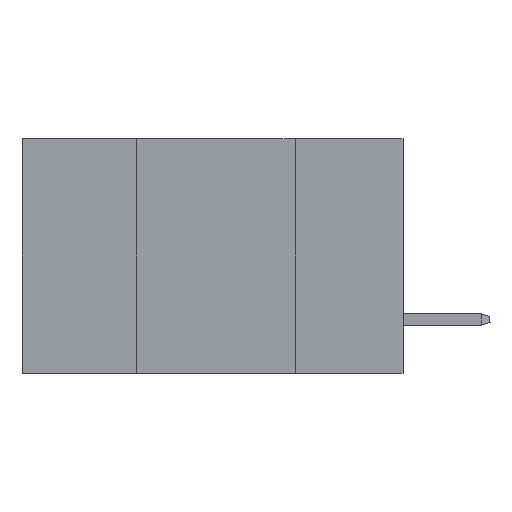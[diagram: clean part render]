
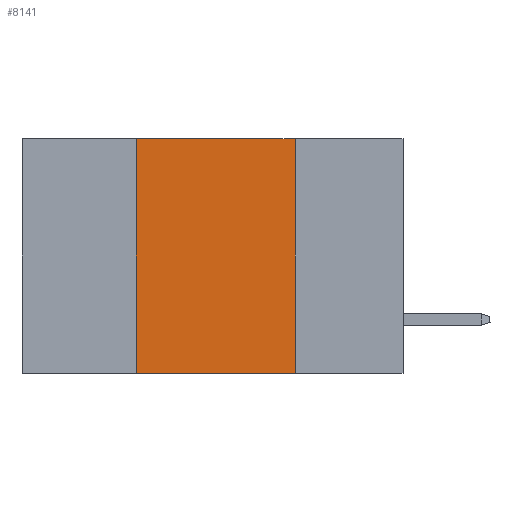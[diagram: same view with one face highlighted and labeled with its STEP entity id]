
A CAD part, left-side view. The second image highlights one B-rep face of the part: STEP entity #8141.
In plain terms, the highlighted planar face has unit normal (-1, 0, 0).
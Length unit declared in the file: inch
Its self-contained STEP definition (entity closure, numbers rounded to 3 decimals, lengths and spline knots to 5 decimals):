
#665 = VECTOR ( 'NONE', #13908, 39.37008 ) ;
#1241 = CARTESIAN_POINT ( 'NONE',  ( 0., 0.6, -0.37 ) ) ;
#1334 = LINE ( 'NONE', #2903, #665 ) ;
#1686 = DIRECTION ( 'NONE',  ( 0., 0., -1. ) ) ;
#1726 = VECTOR ( 'NONE', #15344, 39.37008 ) ;
#2518 = LINE ( 'NONE', #16546, #1726 ) ;
#2889 = ORIENTED_EDGE ( 'NONE', *, *, #7016, .F. ) ;
#2903 = CARTESIAN_POINT ( 'NONE',  ( 0., 0.17, 0. ) ) ;
#3284 = VERTEX_POINT ( 'NONE', #8043 ) ;
#3734 = LINE ( 'NONE', #1241, #16797 ) ;
#3743 = CARTESIAN_POINT ( 'NONE',  ( 0., 0.42, -0.37 ) ) ;
#4167 = VECTOR ( 'NONE', #9340, 39.37008 ) ;
#4375 = PLANE ( 'NONE',  #14692 ) ;
#4532 = ORIENTED_EDGE ( 'NONE', *, *, #15159, .F. ) ;
#6389 = CARTESIAN_POINT ( 'NONE',  ( 0., 0.17, -0.37 ) ) ;
#7016 = EDGE_CURVE ( 'NONE', #3284, #15918, #2518, .T. ) ;
#7417 = CARTESIAN_POINT ( 'NONE',  ( 0., 0.6, 0. ) ) ;
#7606 = FACE_OUTER_BOUND ( 'NONE', #8323, .T. ) ;
#8043 = CARTESIAN_POINT ( 'NONE',  ( 0., 0.42, 0. ) ) ;
#8141 = ADVANCED_FACE ( 'NONE', ( #7606 ), #4375, .F. ) ;
#8297 = VERTEX_POINT ( 'NONE', #6389 ) ;
#8323 = EDGE_LOOP ( 'NONE', ( #4532, #2889, #14118, #9385 ) ) ;
#9154 = LINE ( 'NONE', #14767, #4167 ) ;
#9340 = DIRECTION ( 'NONE',  ( 0., 0., 1. ) ) ;
#9385 = ORIENTED_EDGE ( 'NONE', *, *, #9612, .T. ) ;
#9612 = EDGE_CURVE ( 'NONE', #16180, #8297, #3734, .T. ) ;
#9722 = CARTESIAN_POINT ( 'NONE',  ( 0., 0.17, 0. ) ) ;
#10020 = DIRECTION ( 'NONE',  ( 1., 0., 0. ) ) ;
#11874 = EDGE_CURVE ( 'NONE', #16180, #3284, #9154, .T. ) ;
#13908 = DIRECTION ( 'NONE',  ( 0., 0., -1. ) ) ;
#14118 = ORIENTED_EDGE ( 'NONE', *, *, #11874, .F. ) ;
#14692 = AXIS2_PLACEMENT_3D ( 'NONE', #7417, #10020, #1686 ) ;
#14767 = CARTESIAN_POINT ( 'NONE',  ( 0., 0.42, 0. ) ) ;
#15159 = EDGE_CURVE ( 'NONE', #15918, #8297, #1334, .T. ) ;
#15344 = DIRECTION ( 'NONE',  ( 0., -1., 0. ) ) ;
#15918 = VERTEX_POINT ( 'NONE', #9722 ) ;
#16180 = VERTEX_POINT ( 'NONE', #3743 ) ;
#16546 = CARTESIAN_POINT ( 'NONE',  ( 0., 0.6, 0. ) ) ;
#16674 = DIRECTION ( 'NONE',  ( 0., -1., 0. ) ) ;
#16797 = VECTOR ( 'NONE', #16674, 39.37008 ) ;
